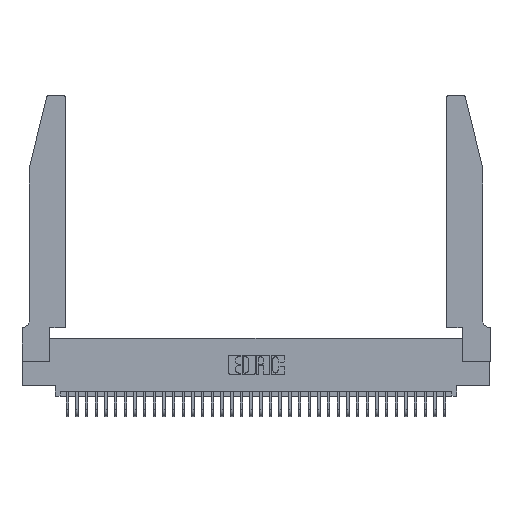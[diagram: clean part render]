
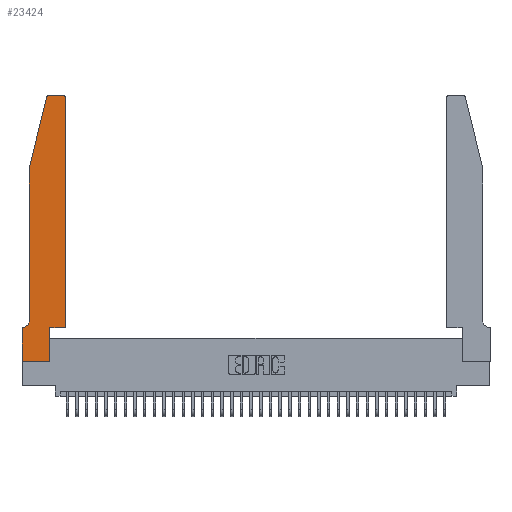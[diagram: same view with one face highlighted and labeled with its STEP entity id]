
A CAD part, top view. The second image highlights one B-rep face of the part: STEP entity #23424.
In plain terms, the highlighted planar face has unit normal (0, 0, 1).
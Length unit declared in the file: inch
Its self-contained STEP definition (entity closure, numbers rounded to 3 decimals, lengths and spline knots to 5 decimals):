
#20 = VERTEX_POINT ( 'NONE', #8065 ) ;
#118 = LINE ( 'NONE', #4224, #3809 ) ;
#211 = EDGE_CURVE ( 'NONE', #36932, #7806, #20559, .T. ) ;
#273 = DIRECTION ( 'NONE',  ( 1., 0., 0. ) ) ;
#772 = CARTESIAN_POINT ( 'NONE',  ( 0., 0.35, 0.37 ) ) ;
#883 = VERTEX_POINT ( 'NONE', #7941 ) ;
#1998 = CARTESIAN_POINT ( 'NONE',  ( 0.4205, 2.75, 0.37 ) ) ;
#2150 = CARTESIAN_POINT ( 'NONE',  ( 0.0055, 0.35, 0.37 ) ) ;
#2576 = ORIENTED_EDGE ( 'NONE', *, *, #15016, .T. ) ;
#2589 = LINE ( 'NONE', #25268, #23780 ) ;
#2701 = VECTOR ( 'NONE', #17988, 39.37008 ) ;
#3249 = CARTESIAN_POINT ( 'NONE',  ( 0.4505, 0.35, 0.37 ) ) ;
#3673 = VERTEX_POINT ( 'NONE', #16502 ) ;
#3809 = VECTOR ( 'NONE', #15951, 39.37008 ) ;
#4187 = CARTESIAN_POINT ( 'NONE',  ( 0., 0., 0.37 ) ) ;
#4224 = CARTESIAN_POINT ( 'NONE',  ( 0.0755, 2., 0.37 ) ) ;
#4712 = EDGE_CURVE ( 'NONE', #5910, #36932, #24788, .T. ) ;
#5299 = DIRECTION ( 'NONE',  ( 1., 0., 0. ) ) ;
#5910 = VERTEX_POINT ( 'NONE', #2150 ) ;
#6638 = LINE ( 'NONE', #11062, #29274 ) ;
#7327 = ORIENTED_EDGE ( 'NONE', *, *, #31828, .T. ) ;
#7632 = LINE ( 'NONE', #17030, #38124 ) ;
#7774 = VECTOR ( 'NONE', #273, 39.37008 ) ;
#7806 = VERTEX_POINT ( 'NONE', #4187 ) ;
#7941 = CARTESIAN_POINT ( 'NONE',  ( 0.284, 2.75, 0.37 ) ) ;
#8065 = CARTESIAN_POINT ( 'NONE',  ( 0.0755, 2., 0.37 ) ) ;
#8590 = EDGE_LOOP ( 'NONE', ( #26200, #17185, #28454, #2576, #15084, #36648, #32111, #10640, #17658, #25758, #7327, #30438 ) ) ;
#9617 = LINE ( 'NONE', #35381, #7774 ) ;
#10377 = CARTESIAN_POINT ( 'NONE',  ( 0., 0.35, 0.37 ) ) ;
#10517 = CIRCLE ( 'NONE', #23249, 0.07 ) ;
#10640 = ORIENTED_EDGE ( 'NONE', *, *, #17905, .T. ) ;
#10998 = LINE ( 'NONE', #19619, #14714 ) ;
#11062 = CARTESIAN_POINT ( 'NONE',  ( 0., 0., 0.37 ) ) ;
#11242 = VERTEX_POINT ( 'NONE', #31259 ) ;
#12294 = CARTESIAN_POINT ( 'NONE',  ( 0.0755, 0.35, 0.37 ) ) ;
#12541 = DIRECTION ( 'NONE',  ( 1., 0., 0. ) ) ;
#12764 = CARTESIAN_POINT ( 'NONE',  ( 0.2865, 0.35, 0.37 ) ) ;
#12766 = VERTEX_POINT ( 'NONE', #30686 ) ;
#14027 = DIRECTION ( 'NONE',  ( 0., 0., -1. ) ) ;
#14164 = CARTESIAN_POINT ( 'NONE',  ( 0.0055, 0.42, 0.37 ) ) ;
#14714 = VECTOR ( 'NONE', #31197, 39.37008 ) ;
#14858 = EDGE_CURVE ( 'NONE', #3673, #33434, #2589, .T. ) ;
#15016 = EDGE_CURVE ( 'NONE', #20, #17440, #7632, .T. ) ;
#15084 = ORIENTED_EDGE ( 'NONE', *, *, #32471, .T. ) ;
#15255 = CARTESIAN_POINT ( 'NONE',  ( 0.2605, 2.75, 0.37 ) ) ;
#15274 = VERTEX_POINT ( 'NONE', #1998 ) ;
#15951 = DIRECTION ( 'NONE',  ( -0.239, -0.971, 0. ) ) ;
#16120 = AXIS2_PLACEMENT_3D ( 'NONE', #22814, #19979, #5299 ) ;
#16502 = CARTESIAN_POINT ( 'NONE',  ( 0.2865, 0., 0.37 ) ) ;
#16987 = VECTOR ( 'NONE', #20963, 39.37008 ) ;
#17030 = CARTESIAN_POINT ( 'NONE',  ( 0.0755, 2., 0.37 ) ) ;
#17185 = ORIENTED_EDGE ( 'NONE', *, *, #31694, .T. ) ;
#17440 = VERTEX_POINT ( 'NONE', #29732 ) ;
#17658 = ORIENTED_EDGE ( 'NONE', *, *, #14858, .T. ) ;
#17905 = EDGE_CURVE ( 'NONE', #7806, #3673, #6638, .T. ) ;
#17988 = DIRECTION ( 'NONE',  ( -1., 0., 0. ) ) ;
#18623 = EDGE_CURVE ( 'NONE', #12766, #20, #118, .T. ) ;
#19284 = AXIS2_PLACEMENT_3D ( 'NONE', #24741, #33376, #27963 ) ;
#19619 = CARTESIAN_POINT ( 'NONE',  ( 0.4505, 0.35, 0.37 ) ) ;
#19979 = DIRECTION ( 'NONE',  ( 0., 0., 1. ) ) ;
#20559 = LINE ( 'NONE', #35870, #36167 ) ;
#20963 = DIRECTION ( 'NONE',  ( -1., 0., 0. ) ) ;
#21259 = EDGE_CURVE ( 'NONE', #11242, #15274, #22571, .T. ) ;
#21469 = PLANE ( 'NONE',  #22875 ) ;
#22028 = EDGE_CURVE ( 'NONE', #33434, #24037, #9617, .T. ) ;
#22571 = CIRCLE ( 'NONE', #16120, 0.03 ) ;
#22814 = CARTESIAN_POINT ( 'NONE',  ( 0.4205, 2.72, 0.37 ) ) ;
#22875 = AXIS2_PLACEMENT_3D ( 'NONE', #772, #33539, #12541 ) ;
#23249 = AXIS2_PLACEMENT_3D ( 'NONE', #14164, #14027, #34645 ) ;
#23424 = ADVANCED_FACE ( 'NONE', ( #36228 ), #21469, .T. ) ;
#23780 = VECTOR ( 'NONE', #27813, 39.37008 ) ;
#23922 = CIRCLE ( 'NONE', #19284, 0.03 ) ;
#24037 = VERTEX_POINT ( 'NONE', #3249 ) ;
#24741 = CARTESIAN_POINT ( 'NONE',  ( 0.284, 2.72, 0.37 ) ) ;
#24788 = LINE ( 'NONE', #12294, #16987 ) ;
#25268 = CARTESIAN_POINT ( 'NONE',  ( 0.2865, 0.35, 0.37 ) ) ;
#25274 = LINE ( 'NONE', #15255, #2701 ) ;
#25758 = ORIENTED_EDGE ( 'NONE', *, *, #22028, .T. ) ;
#25960 = DIRECTION ( 'NONE',  ( 0., -1., 0. ) ) ;
#26200 = ORIENTED_EDGE ( 'NONE', *, *, #36376, .T. ) ;
#27813 = DIRECTION ( 'NONE',  ( 0., 1., 0. ) ) ;
#27963 = DIRECTION ( 'NONE',  ( 1., 0., 0. ) ) ;
#28454 = ORIENTED_EDGE ( 'NONE', *, *, #18623, .T. ) ;
#29274 = VECTOR ( 'NONE', #37617, 39.37008 ) ;
#29732 = CARTESIAN_POINT ( 'NONE',  ( 0.0755, 0.42, 0.37 ) ) ;
#29934 = DIRECTION ( 'NONE',  ( 0., -1., 0. ) ) ;
#30438 = ORIENTED_EDGE ( 'NONE', *, *, #21259, .T. ) ;
#30686 = CARTESIAN_POINT ( 'NONE',  ( 0.25487, 2.72718, 0.37 ) ) ;
#31197 = DIRECTION ( 'NONE',  ( 0., 1., 0. ) ) ;
#31259 = CARTESIAN_POINT ( 'NONE',  ( 0.4505, 2.72, 0.37 ) ) ;
#31694 = EDGE_CURVE ( 'NONE', #883, #12766, #23922, .T. ) ;
#31828 = EDGE_CURVE ( 'NONE', #24037, #11242, #10998, .T. ) ;
#32111 = ORIENTED_EDGE ( 'NONE', *, *, #211, .T. ) ;
#32471 = EDGE_CURVE ( 'NONE', #17440, #5910, #10517, .T. ) ;
#33376 = DIRECTION ( 'NONE',  ( 0., 0., 1. ) ) ;
#33434 = VERTEX_POINT ( 'NONE', #12764 ) ;
#33539 = DIRECTION ( 'NONE',  ( 0., 0., 1. ) ) ;
#34645 = DIRECTION ( 'NONE',  ( -1., 0., 0. ) ) ;
#35381 = CARTESIAN_POINT ( 'NONE',  ( 0.4505, 0.35, 0.37 ) ) ;
#35870 = CARTESIAN_POINT ( 'NONE',  ( 0., 0., 0.37 ) ) ;
#36167 = VECTOR ( 'NONE', #29934, 39.37008 ) ;
#36228 = FACE_OUTER_BOUND ( 'NONE', #8590, .T. ) ;
#36376 = EDGE_CURVE ( 'NONE', #15274, #883, #25274, .T. ) ;
#36648 = ORIENTED_EDGE ( 'NONE', *, *, #4712, .T. ) ;
#36932 = VERTEX_POINT ( 'NONE', #10377 ) ;
#37617 = DIRECTION ( 'NONE',  ( 1., 0., 0. ) ) ;
#38124 = VECTOR ( 'NONE', #25960, 39.37008 ) ;
